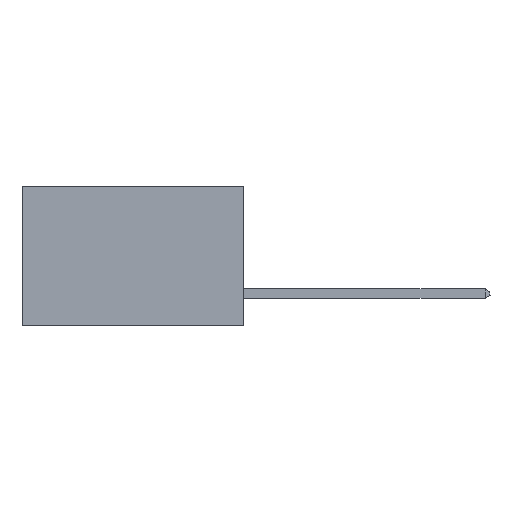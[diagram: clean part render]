
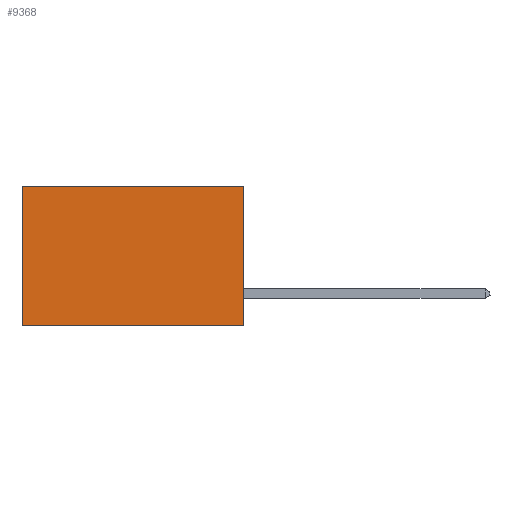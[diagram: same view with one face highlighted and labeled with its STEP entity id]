
A CAD part, left-side view. The second image highlights one B-rep face of the part: STEP entity #9368.
In plain terms, the highlighted planar face has unit normal (-1, 0, 0).
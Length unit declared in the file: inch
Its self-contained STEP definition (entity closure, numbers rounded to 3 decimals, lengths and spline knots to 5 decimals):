
#195 = CARTESIAN_POINT ( 'NONE',  ( 0.277, 0., -0.37 ) ) ;
#450 = EDGE_CURVE ( 'NONE', #13979, #18814, #13279, .T. ) ;
#812 = PLANE ( 'NONE',  #3003 ) ;
#1100 = VECTOR ( 'NONE', #10937, 39.37008 ) ;
#2601 = VECTOR ( 'NONE', #18066, 39.37008 ) ;
#3003 = AXIS2_PLACEMENT_3D ( 'NONE', #3174, #18100, #5309 ) ;
#3060 = VECTOR ( 'NONE', #4321, 39.37008 ) ;
#3142 = VERTEX_POINT ( 'NONE', #8906 ) ;
#3174 = CARTESIAN_POINT ( 'NONE',  ( 0.277, 0., -0.37 ) ) ;
#3331 = EDGE_LOOP ( 'NONE', ( #15485, #21817, #5136, #24151 ) ) ;
#4321 = DIRECTION ( 'NONE',  ( 0., 1., 0. ) ) ;
#4440 = DIRECTION ( 'NONE',  ( 0., 0., -1. ) ) ;
#5136 = ORIENTED_EDGE ( 'NONE', *, *, #20521, .F. ) ;
#5159 = CARTESIAN_POINT ( 'NONE',  ( 0.277, 0., -0.37 ) ) ;
#5309 = DIRECTION ( 'NONE',  ( 0., 0., -1. ) ) ;
#8650 = LINE ( 'NONE', #27646, #3060 ) ;
#8906 = CARTESIAN_POINT ( 'NONE',  ( 0.277, 0.59, -0.37 ) ) ;
#9368 = ADVANCED_FACE ( 'NONE', ( #17411 ), #812, .F. ) ;
#10937 = DIRECTION ( 'NONE',  ( 0., 0., -1. ) ) ;
#13038 = CARTESIAN_POINT ( 'NONE',  ( 0.277, 0., 0. ) ) ;
#13279 = LINE ( 'NONE', #13038, #2601 ) ;
#13345 = VERTEX_POINT ( 'NONE', #5159 ) ;
#13979 = VERTEX_POINT ( 'NONE', #22222 ) ;
#14766 = VECTOR ( 'NONE', #4440, 39.37008 ) ;
#15485 = ORIENTED_EDGE ( 'NONE', *, *, #23606, .T. ) ;
#17411 = FACE_OUTER_BOUND ( 'NONE', #3331, .T. ) ;
#18066 = DIRECTION ( 'NONE',  ( 0., 1., 0. ) ) ;
#18100 = DIRECTION ( 'NONE',  ( 1., 0., 0. ) ) ;
#18230 = LINE ( 'NONE', #195, #1100 ) ;
#18814 = VERTEX_POINT ( 'NONE', #20719 ) ;
#19286 = CARTESIAN_POINT ( 'NONE',  ( 0.277, 0.59, -0.37 ) ) ;
#20521 = EDGE_CURVE ( 'NONE', #13979, #13345, #18230, .T. ) ;
#20719 = CARTESIAN_POINT ( 'NONE',  ( 0.277, 0.59, 0. ) ) ;
#21817 = ORIENTED_EDGE ( 'NONE', *, *, #24267, .F. ) ;
#22222 = CARTESIAN_POINT ( 'NONE',  ( 0.277, 0., 0. ) ) ;
#23606 = EDGE_CURVE ( 'NONE', #18814, #3142, #27372, .T. ) ;
#24151 = ORIENTED_EDGE ( 'NONE', *, *, #450, .T. ) ;
#24267 = EDGE_CURVE ( 'NONE', #13345, #3142, #8650, .T. ) ;
#27372 = LINE ( 'NONE', #19286, #14766 ) ;
#27646 = CARTESIAN_POINT ( 'NONE',  ( 0.277, 0., -0.37 ) ) ;
